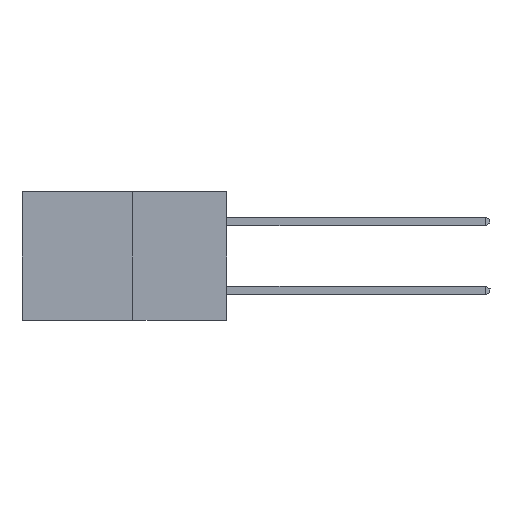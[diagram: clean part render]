
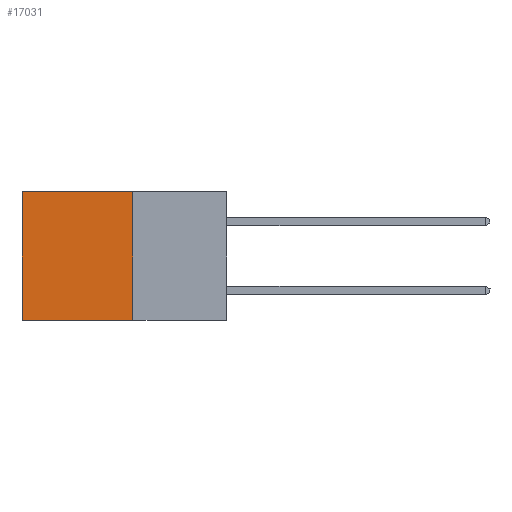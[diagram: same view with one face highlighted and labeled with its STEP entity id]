
A CAD part, left-side view. The second image highlights one B-rep face of the part: STEP entity #17031.
In plain terms, the highlighted planar face has unit normal (-1, 0, 0).
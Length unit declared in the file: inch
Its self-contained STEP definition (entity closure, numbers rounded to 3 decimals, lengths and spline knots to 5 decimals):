
#2132 = PLANE ( 'NONE',  #12209 ) ;
#4618 = EDGE_LOOP ( 'NONE', ( #27723, #7853, #9788, #9636 ) ) ;
#4908 = CARTESIAN_POINT ( 'NONE',  ( 0.277, 0.27, -0.37 ) ) ;
#6313 = EDGE_CURVE ( 'NONE', #9817, #28619, #6948, .T. ) ;
#6875 = DIRECTION ( 'NONE',  ( 0., 0., -1. ) ) ;
#6948 = LINE ( 'NONE', #13120, #12338 ) ;
#7142 = VERTEX_POINT ( 'NONE', #16327 ) ;
#7853 = ORIENTED_EDGE ( 'NONE', *, *, #16296, .F. ) ;
#9636 = ORIENTED_EDGE ( 'NONE', *, *, #6313, .T. ) ;
#9788 = ORIENTED_EDGE ( 'NONE', *, *, #29793, .F. ) ;
#9817 = VERTEX_POINT ( 'NONE', #14302 ) ;
#10107 = VECTOR ( 'NONE', #15929, 39.37008 ) ;
#12209 = AXIS2_PLACEMENT_3D ( 'NONE', #18357, #20677, #6875 ) ;
#12338 = VECTOR ( 'NONE', #26948, 39.37008 ) ;
#13120 = CARTESIAN_POINT ( 'NONE',  ( 0.277, 0.27, 0. ) ) ;
#13505 = VECTOR ( 'NONE', #19429, 39.37008 ) ;
#13982 = DIRECTION ( 'NONE',  ( 0., 1., 0. ) ) ;
#14233 = LINE ( 'NONE', #23970, #13505 ) ;
#14302 = CARTESIAN_POINT ( 'NONE',  ( 0.277, 0.27, 0. ) ) ;
#15929 = DIRECTION ( 'NONE',  ( 0., 0., -1. ) ) ;
#16296 = EDGE_CURVE ( 'NONE', #23726, #7142, #29426, .T. ) ;
#16327 = CARTESIAN_POINT ( 'NONE',  ( 0.277, 0.59, -0.37 ) ) ;
#16482 = VECTOR ( 'NONE', #13982, 39.37008 ) ;
#17031 = ADVANCED_FACE ( 'NONE', ( #17340 ), #2132, .F. ) ;
#17306 = EDGE_CURVE ( 'NONE', #28619, #7142, #14233, .T. ) ;
#17340 = FACE_OUTER_BOUND ( 'NONE', #4618, .T. ) ;
#18300 = CARTESIAN_POINT ( 'NONE',  ( 0.277, 0.59, 0. ) ) ;
#18357 = CARTESIAN_POINT ( 'NONE',  ( 0.277, 0.27, -0.37 ) ) ;
#19429 = DIRECTION ( 'NONE',  ( 0., 0., -1. ) ) ;
#20677 = DIRECTION ( 'NONE',  ( 1., 0., 0. ) ) ;
#23726 = VERTEX_POINT ( 'NONE', #29928 ) ;
#23970 = CARTESIAN_POINT ( 'NONE',  ( 0.277, 0.59, -0.37 ) ) ;
#26948 = DIRECTION ( 'NONE',  ( 0., 1., 0. ) ) ;
#27318 = CARTESIAN_POINT ( 'NONE',  ( 0.277, 0.27, -0.37 ) ) ;
#27723 = ORIENTED_EDGE ( 'NONE', *, *, #17306, .T. ) ;
#28619 = VERTEX_POINT ( 'NONE', #18300 ) ;
#29223 = LINE ( 'NONE', #27318, #10107 ) ;
#29426 = LINE ( 'NONE', #4908, #16482 ) ;
#29793 = EDGE_CURVE ( 'NONE', #9817, #23726, #29223, .T. ) ;
#29928 = CARTESIAN_POINT ( 'NONE',  ( 0.277, 0.27, -0.37 ) ) ;
